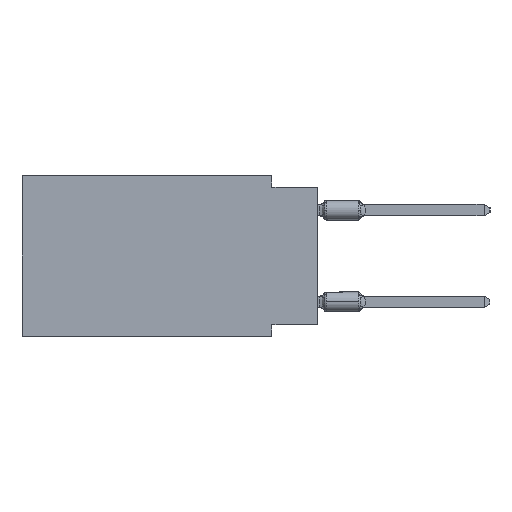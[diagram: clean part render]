
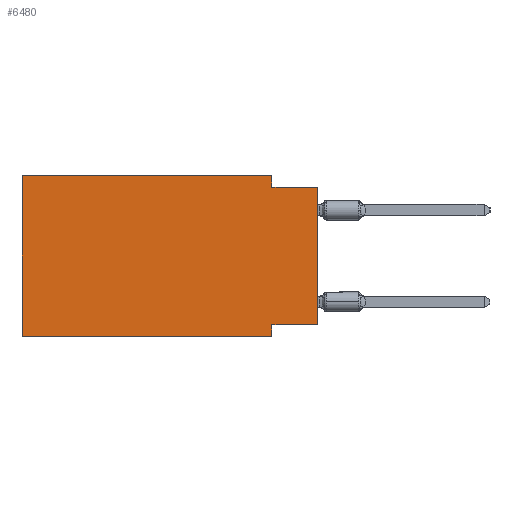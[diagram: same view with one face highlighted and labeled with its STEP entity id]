
A CAD part, left-side view. The second image highlights one B-rep face of the part: STEP entity #6480.
In plain terms, the highlighted planar face has unit normal (-1, 0, 0).
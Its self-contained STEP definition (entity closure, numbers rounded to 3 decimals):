
#1144 = LINE ( 'NONE', #26616, #1843 ) ;
#1605 = CARTESIAN_POINT ( 'NONE',  ( 0., 16.383, 0. ) ) ;
#1664 = FACE_OUTER_BOUND ( 'NONE', #15698, .T. ) ;
#1843 = VECTOR ( 'NONE', #8719, 1000. ) ;
#1943 = AXIS2_PLACEMENT_3D ( 'NONE', #27824, #23924, #46429 ) ;
#3351 = LINE ( 'NONE', #21709, #26309 ) ;
#4720 = VECTOR ( 'NONE', #28941, 1000. ) ;
#5356 = ORIENTED_EDGE ( 'NONE', *, *, #47147, .F. ) ;
#5738 = DIRECTION ( 'NONE',  ( 0., 0., 1. ) ) ;
#6480 = ADVANCED_FACE ( 'NONE', ( #1664 ), #16569, .F. ) ;
#7118 = CARTESIAN_POINT ( 'NONE',  ( 0., 16.383, 0. ) ) ;
#7978 = EDGE_CURVE ( 'NONE', #46924, #27617, #20382, .T. ) ;
#8281 = VECTOR ( 'NONE', #43117, 1000. ) ;
#8395 = VECTOR ( 'NONE', #38180, 1000. ) ;
#8524 = EDGE_CURVE ( 'NONE', #23186, #27617, #3351, .T. ) ;
#8719 = DIRECTION ( 'NONE',  ( 0., 1., 0. ) ) ;
#9438 = ORIENTED_EDGE ( 'NONE', *, *, #22079, .F. ) ;
#9803 = EDGE_CURVE ( 'NONE', #46924, #42434, #1144, .T. ) ;
#9889 = LINE ( 'NONE', #1605, #12227 ) ;
#11286 = LINE ( 'NONE', #23272, #8395 ) ;
#11348 = CARTESIAN_POINT ( 'NONE',  ( 0., 16.383, -8.89 ) ) ;
#12227 = VECTOR ( 'NONE', #5738, 1000. ) ;
#12417 = CARTESIAN_POINT ( 'NONE',  ( 0., 2.54, 0. ) ) ;
#13338 = ORIENTED_EDGE ( 'NONE', *, *, #9803, .F. ) ;
#14026 = CARTESIAN_POINT ( 'NONE',  ( 0., 2.54, -8.89 ) ) ;
#14131 = CARTESIAN_POINT ( 'NONE',  ( 0., 2.54, -0.635 ) ) ;
#15698 = EDGE_LOOP ( 'NONE', ( #38092, #34619, #9438, #5356, #42117, #47245, #42329, #13338 ) ) ;
#16505 = EDGE_CURVE ( 'NONE', #45635, #28358, #9889, .T. ) ;
#16569 = PLANE ( 'NONE',  #1943 ) ;
#19180 = DIRECTION ( 'NONE',  ( 0., -1., 0. ) ) ;
#20382 = LINE ( 'NONE', #38460, #8281 ) ;
#20401 = CARTESIAN_POINT ( 'NONE',  ( 0., 0., -8.255 ) ) ;
#21709 = CARTESIAN_POINT ( 'NONE',  ( 0., 0., -0.635 ) ) ;
#22079 = EDGE_CURVE ( 'NONE', #25242, #23186, #28312, .T. ) ;
#23186 = VERTEX_POINT ( 'NONE', #14131 ) ;
#23272 = CARTESIAN_POINT ( 'NONE',  ( 0., 16.383, 0. ) ) ;
#23924 = DIRECTION ( 'NONE',  ( 1., 0., 0. ) ) ;
#25242 = VERTEX_POINT ( 'NONE', #25557 ) ;
#25557 = CARTESIAN_POINT ( 'NONE',  ( 0., 2.54, 0. ) ) ;
#26309 = VECTOR ( 'NONE', #37336, 1000. ) ;
#26616 = CARTESIAN_POINT ( 'NONE',  ( 0., 0., -8.255 ) ) ;
#26763 = LINE ( 'NONE', #11348, #35511 ) ;
#27617 = VERTEX_POINT ( 'NONE', #46859 ) ;
#27824 = CARTESIAN_POINT ( 'NONE',  ( 0., 16.383, 0. ) ) ;
#28312 = LINE ( 'NONE', #12417, #46939 ) ;
#28358 = VERTEX_POINT ( 'NONE', #7118 ) ;
#28941 = DIRECTION ( 'NONE',  ( 0., 0., -1. ) ) ;
#31064 = EDGE_CURVE ( 'NONE', #45635, #31310, #26763, .T. ) ;
#31310 = VERTEX_POINT ( 'NONE', #43373 ) ;
#34619 = ORIENTED_EDGE ( 'NONE', *, *, #8524, .F. ) ;
#34693 = DIRECTION ( 'NONE',  ( 0., 0., -1. ) ) ;
#35157 = CARTESIAN_POINT ( 'NONE',  ( 0., 2.54, -8.255 ) ) ;
#35511 = VECTOR ( 'NONE', #19180, 1000. ) ;
#35786 = CARTESIAN_POINT ( 'NONE',  ( 0., 16.383, -8.89 ) ) ;
#37336 = DIRECTION ( 'NONE',  ( 0., -1., 0. ) ) ;
#38092 = ORIENTED_EDGE ( 'NONE', *, *, #7978, .T. ) ;
#38180 = DIRECTION ( 'NONE',  ( 0., -1., 0. ) ) ;
#38460 = CARTESIAN_POINT ( 'NONE',  ( 0., 0., 0. ) ) ;
#42117 = ORIENTED_EDGE ( 'NONE', *, *, #16505, .F. ) ;
#42329 = ORIENTED_EDGE ( 'NONE', *, *, #48246, .F. ) ;
#42434 = VERTEX_POINT ( 'NONE', #35157 ) ;
#43117 = DIRECTION ( 'NONE',  ( 0., 0., 1. ) ) ;
#43373 = CARTESIAN_POINT ( 'NONE',  ( 0., 2.54, -8.89 ) ) ;
#45635 = VERTEX_POINT ( 'NONE', #35786 ) ;
#46429 = DIRECTION ( 'NONE',  ( 0., 0., -1. ) ) ;
#46859 = CARTESIAN_POINT ( 'NONE',  ( 0., 0., -0.635 ) ) ;
#46924 = VERTEX_POINT ( 'NONE', #20401 ) ;
#46939 = VECTOR ( 'NONE', #34693, 1000. ) ;
#47147 = EDGE_CURVE ( 'NONE', #28358, #25242, #11286, .T. ) ;
#47245 = ORIENTED_EDGE ( 'NONE', *, *, #31064, .T. ) ;
#47540 = LINE ( 'NONE', #14026, #4720 ) ;
#48246 = EDGE_CURVE ( 'NONE', #42434, #31310, #47540, .T. ) ;
